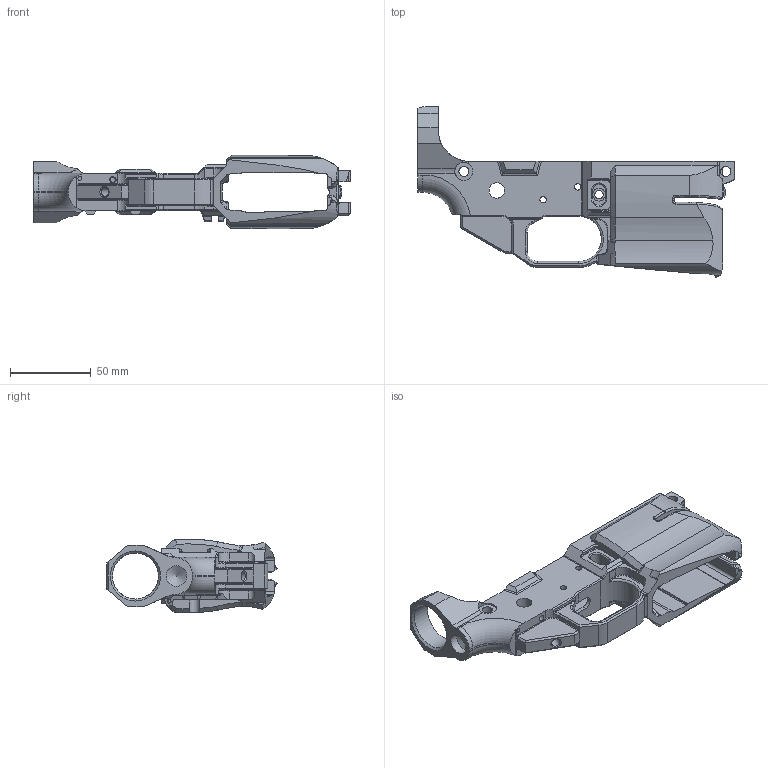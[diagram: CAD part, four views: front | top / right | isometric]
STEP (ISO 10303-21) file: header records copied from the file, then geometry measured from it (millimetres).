
FILE_DESCRIPTION(/* description */ (''),/* implementation_level */ '2;1');
FILE_NAME(/* name */ 'Mando15 v2.step',/* time_stamp */ '2020-09-04T08:42:27-04:00',/* author */ (''),/* organization */ (''),/* preprocessor_version */ 'ST-DEVELOPER v18.1',/* originating_system */ 'Autodesk Translation Framework v9.3.0.1241',/* authorisation */ '');
FILE_SCHEMA (('AUTOMOTIVE_DESIGN { 1 0 10303 214 3 1 1 }'));
Length unit declared in the file: millimetre
Products named in the file (1): Mando15
Bounding box: 195.97 x 105.3 x 45.64 mm (x, y, z)
Volume: 150473.3 mm3; surface area: 62356.9 mm2
Topology: 1 solids, 1 shells, 773 faces, 2136 edges, 1369 vertices
Faces by surface type: plane 366, cylinder 246, bspline 99, cone 42, torus 20
Full cylindrical faces by diameter (mm): 1.985 x1, 2.362 x2, 2.464 x2, 3.175 x1, 3.962 x4, 3.969 x2, 5.182 x1, 5.41 x1, 6.248 x2, 6.375 x2, 6.477 x1, 7.925 x1, 9.55 x2, 11.176 x1, 12.7 x1, 28.448 x1
Entity records: 31151 total; most frequent: CARTESIAN_POINT 11977, ORIENTED_EDGE 4264, DIRECTION 3663, EDGE_CURVE 2132, VERTEX_POINT 1369, AXIS2_PLACEMENT_3D 1240, LINE 1183, VECTOR 1183
